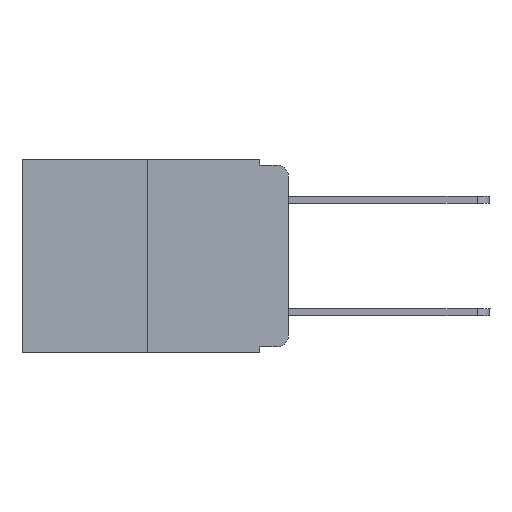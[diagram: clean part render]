
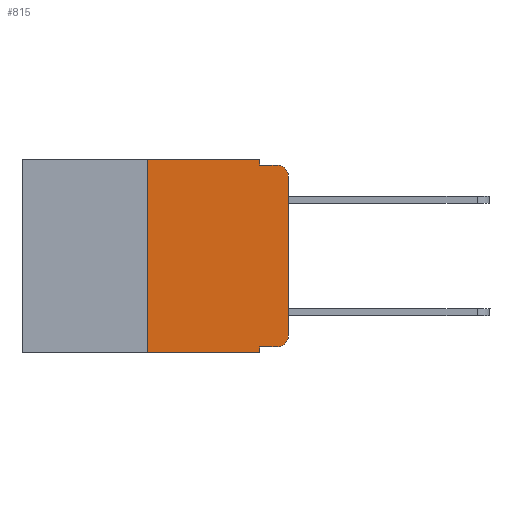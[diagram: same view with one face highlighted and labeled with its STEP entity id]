
A CAD part, left-side view. The second image highlights one B-rep face of the part: STEP entity #815.
In plain terms, the highlighted planar face has unit normal (-1, 0, 0).
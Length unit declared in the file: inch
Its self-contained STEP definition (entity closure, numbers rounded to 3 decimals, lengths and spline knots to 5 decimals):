
#282 = AXIS2_PLACEMENT_3D ( 'NONE', #3602, #16477, #14126 ) ;
#521 = DIRECTION ( 'NONE',  ( 0., 0., -1. ) ) ;
#698 = LINE ( 'NONE', #15296, #6094 ) ;
#815 = ADVANCED_FACE ( 'NONE', ( #11721 ), #16663, .F. ) ;
#933 = CARTESIAN_POINT ( 'NONE',  ( 0., 0., -0.03 ) ) ;
#1111 = CARTESIAN_POINT ( 'NONE',  ( 0., 0.473, 0. ) ) ;
#1533 = CARTESIAN_POINT ( 'NONE',  ( 0., 0.02, -0.01 ) ) ;
#1711 = CARTESIAN_POINT ( 'NONE',  ( 0., 0.25, -0.343 ) ) ;
#1949 = ORIENTED_EDGE ( 'NONE', *, *, #4349, .F. ) ;
#2154 = ORIENTED_EDGE ( 'NONE', *, *, #10165, .F. ) ;
#2388 = VECTOR ( 'NONE', #16537, 39.37008 ) ;
#2616 = ORIENTED_EDGE ( 'NONE', *, *, #13484, .T. ) ;
#2788 = VECTOR ( 'NONE', #12352, 39.37008 ) ;
#3037 = EDGE_CURVE ( 'NONE', #9884, #13555, #7720, .T. ) ;
#3104 = VERTEX_POINT ( 'NONE', #933 ) ;
#3219 = CARTESIAN_POINT ( 'NONE',  ( 0., 0.051, -0.01 ) ) ;
#3397 = LINE ( 'NONE', #12800, #10668 ) ;
#3420 = LINE ( 'NONE', #6172, #2388 ) ;
#3602 = CARTESIAN_POINT ( 'NONE',  ( 0., 0.02, -0.313 ) ) ;
#3642 = VERTEX_POINT ( 'NONE', #15592 ) ;
#3759 = VERTEX_POINT ( 'NONE', #16262 ) ;
#3920 = EDGE_CURVE ( 'NONE', #6203, #9991, #4857, .T. ) ;
#4349 = EDGE_CURVE ( 'NONE', #3642, #9991, #698, .T. ) ;
#4596 = EDGE_CURVE ( 'NONE', #3642, #9884, #5415, .T. ) ;
#4675 = DIRECTION ( 'NONE',  ( 0., 0., -1. ) ) ;
#4857 = LINE ( 'NONE', #12531, #2788 ) ;
#5282 = VERTEX_POINT ( 'NONE', #3219 ) ;
#5324 = ORIENTED_EDGE ( 'NONE', *, *, #3037, .T. ) ;
#5415 = LINE ( 'NONE', #10672, #13284 ) ;
#5429 = CARTESIAN_POINT ( 'NONE',  ( 0., 0.25, 0. ) ) ;
#5510 = DIRECTION ( 'NONE',  ( 0., 0., 1. ) ) ;
#5629 = LINE ( 'NONE', #5777, #9958 ) ;
#5777 = CARTESIAN_POINT ( 'NONE',  ( 0., 0.473, 0. ) ) ;
#5898 = ORIENTED_EDGE ( 'NONE', *, *, #13933, .F. ) ;
#6094 = VECTOR ( 'NONE', #521, 39.37008 ) ;
#6172 = CARTESIAN_POINT ( 'NONE',  ( 0., 0., 0. ) ) ;
#6188 = EDGE_CURVE ( 'NONE', #6203, #12051, #8353, .T. ) ;
#6203 = VERTEX_POINT ( 'NONE', #1711 ) ;
#7328 = ORIENTED_EDGE ( 'NONE', *, *, #14948, .F. ) ;
#7518 = ORIENTED_EDGE ( 'NONE', *, *, #6188, .F. ) ;
#7670 = DIRECTION ( 'NONE',  ( 0., -1., 0. ) ) ;
#7720 = CIRCLE ( 'NONE', #282, 0.02 ) ;
#7897 = CARTESIAN_POINT ( 'NONE',  ( 0., 0.02, -0.03 ) ) ;
#8353 = LINE ( 'NONE', #5429, #12770 ) ;
#8709 = DIRECTION ( 'NONE',  ( 0., 0., -1. ) ) ;
#8875 = DIRECTION ( 'NONE',  ( 1., 0., 0. ) ) ;
#9048 = ORIENTED_EDGE ( 'NONE', *, *, #16040, .T. ) ;
#9114 = DIRECTION ( 'NONE',  ( 0., 0., -1. ) ) ;
#9378 = DIRECTION ( 'NONE',  ( 0., -1., 0. ) ) ;
#9696 = AXIS2_PLACEMENT_3D ( 'NONE', #7897, #14375, #9114 ) ;
#9884 = VERTEX_POINT ( 'NONE', #11423 ) ;
#9958 = VECTOR ( 'NONE', #16331, 39.37008 ) ;
#9979 = CIRCLE ( 'NONE', #9696, 0.02 ) ;
#9991 = VERTEX_POINT ( 'NONE', #15831 ) ;
#10165 = EDGE_CURVE ( 'NONE', #5282, #16215, #13470, .T. ) ;
#10668 = VECTOR ( 'NONE', #4675, 39.37008 ) ;
#10672 = CARTESIAN_POINT ( 'NONE',  ( 0., 0.051, -0.333 ) ) ;
#11169 = CARTESIAN_POINT ( 'NONE',  ( 0., 0.25, 0. ) ) ;
#11423 = CARTESIAN_POINT ( 'NONE',  ( 0., 0.02, -0.333 ) ) ;
#11721 = FACE_OUTER_BOUND ( 'NONE', #14044, .T. ) ;
#12051 = VERTEX_POINT ( 'NONE', #11169 ) ;
#12352 = DIRECTION ( 'NONE',  ( 0., -1., 0. ) ) ;
#12451 = ORIENTED_EDGE ( 'NONE', *, *, #4596, .T. ) ;
#12531 = CARTESIAN_POINT ( 'NONE',  ( 0., 0.473, -0.343 ) ) ;
#12770 = VECTOR ( 'NONE', #5510, 39.37008 ) ;
#12800 = CARTESIAN_POINT ( 'NONE',  ( 0., 0.051, 0. ) ) ;
#12816 = CARTESIAN_POINT ( 'NONE',  ( 0., 0., -0.313 ) ) ;
#12888 = ORIENTED_EDGE ( 'NONE', *, *, #3920, .T. ) ;
#13086 = VECTOR ( 'NONE', #7670, 39.37008 ) ;
#13284 = VECTOR ( 'NONE', #9378, 39.37008 ) ;
#13470 = LINE ( 'NONE', #16834, #13086 ) ;
#13484 = EDGE_CURVE ( 'NONE', #13555, #3104, #3420, .T. ) ;
#13555 = VERTEX_POINT ( 'NONE', #12816 ) ;
#13917 = AXIS2_PLACEMENT_3D ( 'NONE', #1111, #8875, #8709 ) ;
#13933 = EDGE_CURVE ( 'NONE', #3759, #5282, #3397, .T. ) ;
#14044 = EDGE_LOOP ( 'NONE', ( #2616, #9048, #2154, #5898, #7328, #7518, #12888, #1949, #12451, #5324 ) ) ;
#14126 = DIRECTION ( 'NONE',  ( 0., 0., -1. ) ) ;
#14375 = DIRECTION ( 'NONE',  ( -1., 0., 0. ) ) ;
#14948 = EDGE_CURVE ( 'NONE', #12051, #3759, #5629, .T. ) ;
#15296 = CARTESIAN_POINT ( 'NONE',  ( 0., 0.051, 0. ) ) ;
#15592 = CARTESIAN_POINT ( 'NONE',  ( 0., 0.051, -0.333 ) ) ;
#15831 = CARTESIAN_POINT ( 'NONE',  ( 0., 0.051, -0.343 ) ) ;
#16040 = EDGE_CURVE ( 'NONE', #3104, #16215, #9979, .T. ) ;
#16215 = VERTEX_POINT ( 'NONE', #1533 ) ;
#16262 = CARTESIAN_POINT ( 'NONE',  ( 0., 0.051, 0. ) ) ;
#16331 = DIRECTION ( 'NONE',  ( 0., -1., 0. ) ) ;
#16477 = DIRECTION ( 'NONE',  ( -1., 0., 0. ) ) ;
#16537 = DIRECTION ( 'NONE',  ( 0., 0., 1. ) ) ;
#16663 = PLANE ( 'NONE',  #13917 ) ;
#16834 = CARTESIAN_POINT ( 'NONE',  ( 0., 0.051, -0.01 ) ) ;
